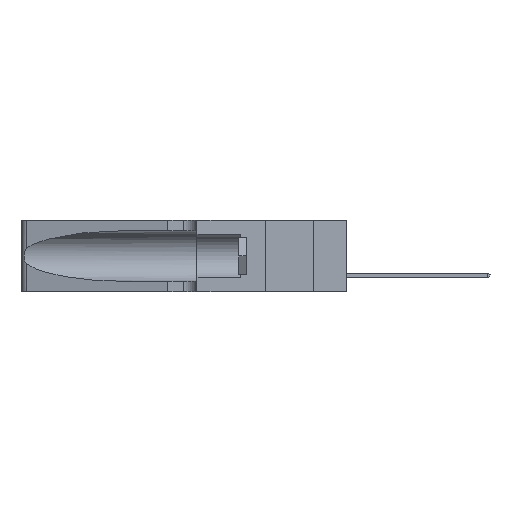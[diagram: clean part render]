
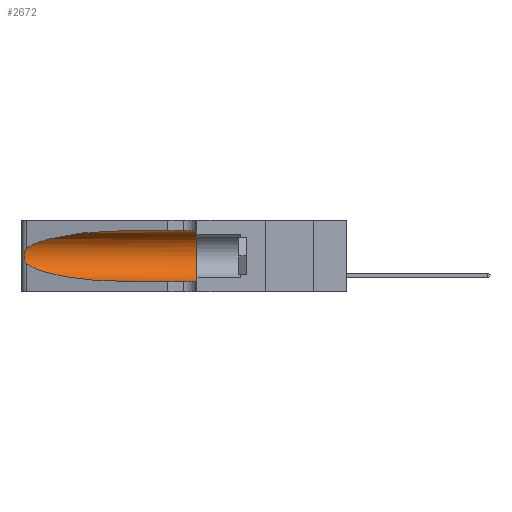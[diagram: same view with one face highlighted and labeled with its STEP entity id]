
A CAD part, left-side view. The second image highlights one B-rep face of the part: STEP entity #2672.
In plain terms, the highlighted cylindrical face has radius 3.308 mm (diameter 6.617 mm), a partial arc.
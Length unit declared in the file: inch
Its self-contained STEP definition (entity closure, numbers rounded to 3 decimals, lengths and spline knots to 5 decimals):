
#807 = DIRECTION ( 'NONE',  ( 0., 0., 1. ) ) ;
#957 = ORIENTED_EDGE ( 'NONE', *, *, #22672, .F. ) ;
#1020 = VERTEX_POINT ( 'NONE', #23946 ) ;
#2094 = CARTESIAN_POINT ( 'NONE',  ( 0.26018, 1.23835, 0.19895 ) ) ;
#2598 = CARTESIAN_POINT ( 'NONE',  ( 0.18966, 0.96281, 0.31525 ) ) ;
#2664 = VERTEX_POINT ( 'NONE', #5445 ) ;
#2672 = ADVANCED_FACE ( 'NONE', ( #40470 ), #37311, .F. ) ;
#3024 = CARTESIAN_POINT ( 'NONE',  ( 0.18966, 0.96281, 0.05475 ) ) ;
#3065 = AXIS2_PLACEMENT_3D ( 'NONE', #11119, #17676, #807 ) ;
#4862 = ORIENTED_EDGE ( 'NONE', *, *, #29958, .T. ) ;
#5438 = EDGE_CURVE ( 'NONE', #29805, #13073, #32112, .T. ) ;
#5445 = CARTESIAN_POINT ( 'NONE',  ( 0.25487, 1.22718, 0.14631 ) ) ;
#5580 = ORIENTED_EDGE ( 'NONE', *, *, #29566, .T. ) ;
#5653 = ORIENTED_EDGE ( 'NONE', *, *, #21653, .F. ) ;
#8818 = EDGE_LOOP ( 'NONE', ( #10185, #4862, #5580, #10963, #5653, #957 ) ) ;
#8831 = CARTESIAN_POINT ( 'NONE',  ( 0.26075, 1.23896, 0.178 ) ) ;
#8974 = CARTESIAN_POINT ( 'NONE',  ( 0.25789, 1.23486, 0.15765 ) ) ;
#9029 = CARTESIAN_POINT ( 'NONE',  ( 0.1305, 0.72297, 0.31525 ) ) ;
#9423 = CARTESIAN_POINT ( 'NONE',  ( 0.1305, 0.35, 0.31525 ) ) ;
#10185 = ORIENTED_EDGE ( 'NONE', *, *, #5438, .T. ) ;
#10963 = ORIENTED_EDGE ( 'NONE', *, *, #13895, .T. ) ;
#11119 = CARTESIAN_POINT ( 'NONE',  ( 0.1305, 0.35, 0.185 ) ) ;
#11166 = CARTESIAN_POINT ( 'NONE',  ( 0.1305, 1.61858, 0.31525 ) ) ;
#11316 = CARTESIAN_POINT ( 'NONE',  ( 0.1305, 0.72297, 0.31525 ) ) ;
#11930 = CARTESIAN_POINT ( 'NONE',  ( 0.25487, 1.22718, 0.22369 ) ) ;
#13073 = VERTEX_POINT ( 'NONE', #40882 ) ;
#13541 = VECTOR ( 'NONE', #17876, 39.37008 ) ;
#13895 = EDGE_CURVE ( 'NONE', #40855, #1020, #41131, .T. ) ;
#15676 = CARTESIAN_POINT ( 'NONE',  ( 0.25856, 1.23593, 0.16098 ) ) ;
#16948 =( BOUNDED_CURVE ( )  B_SPLINE_CURVE ( 3, ( #30354, #20169, #3024, #26711 ),
 .UNSPECIFIED., .F., .F. ) 
 B_SPLINE_CURVE_WITH_KNOTS ( ( 4, 4 ),
 ( 3.44316, 4.71239 ),
 .UNSPECIFIED. ) 
 CURVE ( )  GEOMETRIC_REPRESENTATION_ITEM ( )  RATIONAL_B_SPLINE_CURVE ( ( 1., 0.87, 0.87, 1. ) ) 
 REPRESENTATION_ITEM ( '' )  );
#17676 = DIRECTION ( 'NONE',  ( 0., 1., 0. ) ) ;
#17876 = DIRECTION ( 'NONE',  ( 0., -1., 0. ) ) ;
#18953 = CARTESIAN_POINT ( 'NONE',  ( 0.25787, 1.23484, 0.2124 ) ) ;
#19293 = CARTESIAN_POINT ( 'NONE',  ( 0.25487, 1.22718, 0.22369 ) ) ;
#20003 = LINE ( 'NONE', #11166, #13541 ) ;
#20169 = CARTESIAN_POINT ( 'NONE',  ( 0.2373, 1.15595, 0.08982 ) ) ;
#20254 = DIRECTION ( 'NONE',  ( 0., 0., -1. ) ) ;
#21071 = VECTOR ( 'NONE', #22702, 39.37008 ) ;
#21653 = EDGE_CURVE ( 'NONE', #23445, #1020, #35194, .T. ) ;
#22507 = CARTESIAN_POINT ( 'NONE',  ( 0.26017, 1.23833, 0.17102 ) ) ;
#22672 = EDGE_CURVE ( 'NONE', #29805, #23445, #20003, .T. ) ;
#22702 = DIRECTION ( 'NONE',  ( 0., -1., 0. ) ) ;
#23445 = VERTEX_POINT ( 'NONE', #9423 ) ;
#23526 = CARTESIAN_POINT ( 'NONE',  ( 0.25487, 1.22718, 0.14631 ) ) ;
#23946 = CARTESIAN_POINT ( 'NONE',  ( 0.1305, 0.35, 0.05475 ) ) ;
#25769 = CARTESIAN_POINT ( 'NONE',  ( 0.26075, 1.23896, 0.19203 ) ) ;
#26711 = CARTESIAN_POINT ( 'NONE',  ( 0.1305, 0.72297, 0.05475 ) ) ;
#29566 = EDGE_CURVE ( 'NONE', #2664, #40855, #16948, .T. ) ;
#29805 = VERTEX_POINT ( 'NONE', #11316 ) ;
#29958 = EDGE_CURVE ( 'NONE', #13073, #2664, #40998, .T. ) ;
#30354 = CARTESIAN_POINT ( 'NONE',  ( 0.25487, 1.22718, 0.14631 ) ) ;
#32112 =( BOUNDED_CURVE ( )  B_SPLINE_CURVE ( 3, ( #9029, #2598, #36135, #19293 ),
 .UNSPECIFIED., .F., .F. ) 
 B_SPLINE_CURVE_WITH_KNOTS ( ( 4, 4 ),
 ( 1.5708, 2.84003 ),
 .UNSPECIFIED. ) 
 CURVE ( )  GEOMETRIC_REPRESENTATION_ITEM ( )  RATIONAL_B_SPLINE_CURVE ( ( 1., 0.87, 0.87, 1. ) ) 
 REPRESENTATION_ITEM ( '' )  );
#32699 = CARTESIAN_POINT ( 'NONE',  ( 0.25639, 1.23186, 0.15144 ) ) ;
#35019 = CARTESIAN_POINT ( 'NONE',  ( 0.1305, 0.72297, 0.05475 ) ) ;
#35190 = CARTESIAN_POINT ( 'NONE',  ( 0.1305, 1.61858, 0.05475 ) ) ;
#35194 = CIRCLE ( 'NONE', #3065, 0.13025 ) ;
#35793 = CARTESIAN_POINT ( 'NONE',  ( 0.25639, 1.23184, 0.21858 ) ) ;
#36135 = CARTESIAN_POINT ( 'NONE',  ( 0.2373, 1.15595, 0.28018 ) ) ;
#36520 = DIRECTION ( 'NONE',  ( 0., -1., 0. ) ) ;
#36973 = CARTESIAN_POINT ( 'NONE',  ( 0.25555, 1.22993, 0.14849 ) ) ;
#37095 = CARTESIAN_POINT ( 'NONE',  ( 0.1305, 1.61858, 0.185 ) ) ;
#37311 = CYLINDRICAL_SURFACE ( 'NONE', #40828, 0.13025 ) ;
#39055 = CARTESIAN_POINT ( 'NONE',  ( 0.25555, 1.22994, 0.2215 ) ) ;
#40470 = FACE_OUTER_BOUND ( 'NONE', #8818, .T. ) ;
#40828 = AXIS2_PLACEMENT_3D ( 'NONE', #37095, #36520, #20254 ) ;
#40855 = VERTEX_POINT ( 'NONE', #35019 ) ;
#40882 = CARTESIAN_POINT ( 'NONE',  ( 0.25487, 1.22718, 0.22369 ) ) ;
#40998 = B_SPLINE_CURVE_WITH_KNOTS ( 'NONE', 3,
 ( #11930, #39055, #35793, #18953, #42584, #2094, #25769, #8831, #22507, #15676, #8974, #32699, #36973, #23526 ),
 .UNSPECIFIED., .F., .F.,
 ( 4, 2, 2, 2, 2, 2, 4 ),
 ( 0., 0.00027, 0.00053, 0.00107, 0.0016, 0.00187, 0.00214 ),
 .UNSPECIFIED. ) ;
#41131 = LINE ( 'NONE', #35190, #21071 ) ;
#42584 = CARTESIAN_POINT ( 'NONE',  ( 0.25854, 1.2359, 0.20912 ) ) ;
